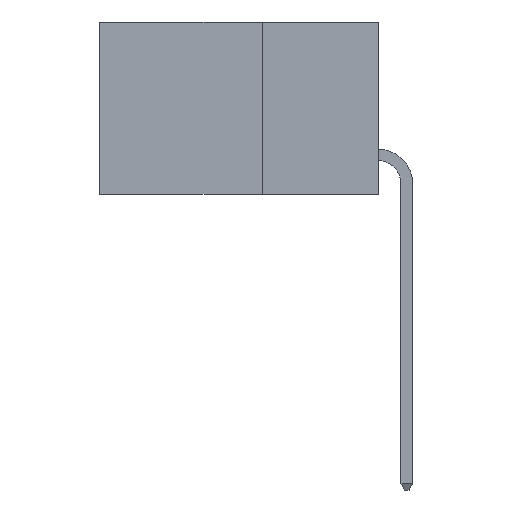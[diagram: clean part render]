
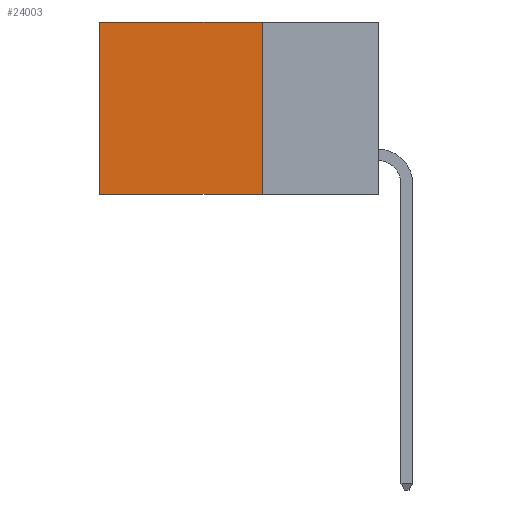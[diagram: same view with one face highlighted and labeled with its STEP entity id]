
A CAD part, left-side view. The second image highlights one B-rep face of the part: STEP entity #24003.
In plain terms, the highlighted planar face has unit normal (-1, 0, 0).
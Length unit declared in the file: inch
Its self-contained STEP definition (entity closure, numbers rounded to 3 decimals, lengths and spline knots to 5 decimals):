
#990 = CARTESIAN_POINT ( 'NONE',  ( 0.2615, 0.25, -0.37 ) ) ;
#1300 = VECTOR ( 'NONE', #17404, 39.37008 ) ;
#1466 = VERTEX_POINT ( 'NONE', #3375 ) ;
#1599 = VERTEX_POINT ( 'NONE', #11299 ) ;
#1945 = ORIENTED_EDGE ( 'NONE', *, *, #21670, .F. ) ;
#1952 = LINE ( 'NONE', #15370, #1300 ) ;
#2417 = EDGE_CURVE ( 'NONE', #1466, #6312, #10325, .T. ) ;
#3343 = DIRECTION ( 'NONE',  ( 0., 0., -1. ) ) ;
#3375 = CARTESIAN_POINT ( 'NONE',  ( 0.2615, 0.25, 0. ) ) ;
#5320 = DIRECTION ( 'NONE',  ( 1., 0., 0. ) ) ;
#6312 = VERTEX_POINT ( 'NONE', #7120 ) ;
#7120 = CARTESIAN_POINT ( 'NONE',  ( 0.2615, 0.6, 0. ) ) ;
#8978 = EDGE_CURVE ( 'NONE', #22240, #1599, #20300, .T. ) ;
#9563 = VECTOR ( 'NONE', #23028, 39.37008 ) ;
#10325 = LINE ( 'NONE', #11597, #19834 ) ;
#10818 = EDGE_LOOP ( 'NONE', ( #18855, #22759, #1945, #19617 ) ) ;
#11017 = DIRECTION ( 'NONE',  ( 0., 1., 0. ) ) ;
#11299 = CARTESIAN_POINT ( 'NONE',  ( 0.2615, 0.6, -0.37 ) ) ;
#11597 = CARTESIAN_POINT ( 'NONE',  ( 0.2615, 0.25, 0. ) ) ;
#13109 = CARTESIAN_POINT ( 'NONE',  ( 0.2615, 0.25, -0.37 ) ) ;
#13572 = CARTESIAN_POINT ( 'NONE',  ( 0.2615, 0.25, -0.37 ) ) ;
#13604 = AXIS2_PLACEMENT_3D ( 'NONE', #13572, #5320, #3343 ) ;
#14958 = VECTOR ( 'NONE', #17389, 39.37008 ) ;
#15370 = CARTESIAN_POINT ( 'NONE',  ( 0.2615, 0.6, -0.37 ) ) ;
#15618 = PLANE ( 'NONE',  #13604 ) ;
#15645 = LINE ( 'NONE', #13109, #9563 ) ;
#17389 = DIRECTION ( 'NONE',  ( 0., 1., 0. ) ) ;
#17404 = DIRECTION ( 'NONE',  ( 0., 0., -1. ) ) ;
#18661 = FACE_OUTER_BOUND ( 'NONE', #10818, .T. ) ;
#18855 = ORIENTED_EDGE ( 'NONE', *, *, #19270, .T. ) ;
#19270 = EDGE_CURVE ( 'NONE', #6312, #1599, #1952, .T. ) ;
#19617 = ORIENTED_EDGE ( 'NONE', *, *, #2417, .T. ) ;
#19834 = VECTOR ( 'NONE', #11017, 39.37008 ) ;
#20300 = LINE ( 'NONE', #990, #14958 ) ;
#21670 = EDGE_CURVE ( 'NONE', #1466, #22240, #15645, .T. ) ;
#22171 = CARTESIAN_POINT ( 'NONE',  ( 0.2615, 0.25, -0.37 ) ) ;
#22240 = VERTEX_POINT ( 'NONE', #22171 ) ;
#22759 = ORIENTED_EDGE ( 'NONE', *, *, #8978, .F. ) ;
#23028 = DIRECTION ( 'NONE',  ( 0., 0., -1. ) ) ;
#24003 = ADVANCED_FACE ( 'NONE', ( #18661 ), #15618, .F. ) ;
